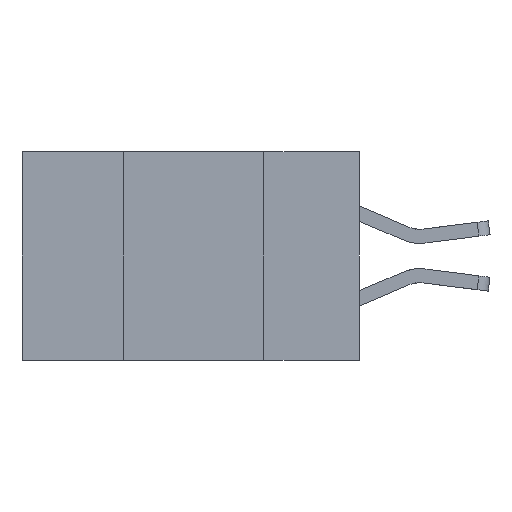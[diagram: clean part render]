
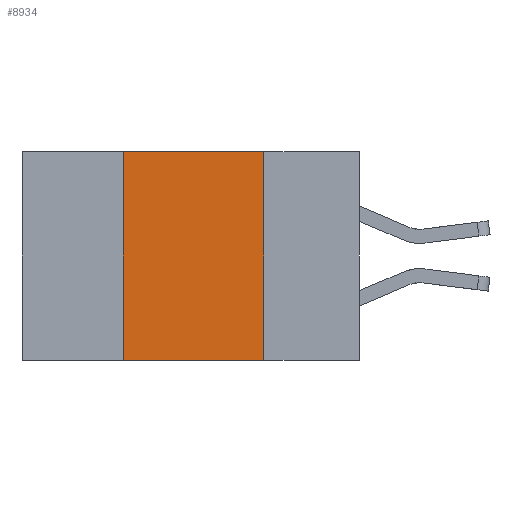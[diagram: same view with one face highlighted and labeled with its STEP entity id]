
A CAD part, left-side view. The second image highlights one B-rep face of the part: STEP entity #8934.
In plain terms, the highlighted planar face has unit normal (-1, 0, 0).
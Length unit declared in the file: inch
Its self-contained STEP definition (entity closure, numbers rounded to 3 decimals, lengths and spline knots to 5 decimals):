
#46 = CARTESIAN_POINT ( 'NONE',  ( 0., 0.42, 0. ) ) ;
#115 = CARTESIAN_POINT ( 'NONE',  ( 0., 0.17, 0. ) ) ;
#658 = CARTESIAN_POINT ( 'NONE',  ( 0., 0.42, 0. ) ) ;
#924 = PLANE ( 'NONE',  #6355 ) ;
#1428 = LINE ( 'NONE', #11579, #11336 ) ;
#2015 = CARTESIAN_POINT ( 'NONE',  ( 0., 0.6, 0. ) ) ;
#2362 = CARTESIAN_POINT ( 'NONE',  ( 0., 0.6, 0. ) ) ;
#2534 = CARTESIAN_POINT ( 'NONE',  ( 0., 0.42, -0.37 ) ) ;
#3047 = DIRECTION ( 'NONE',  ( 1., 0., 0. ) ) ;
#3139 = CARTESIAN_POINT ( 'NONE',  ( 0., 0.17, -0.37 ) ) ;
#3356 = VERTEX_POINT ( 'NONE', #2534 ) ;
#3390 = ORIENTED_EDGE ( 'NONE', *, *, #7328, .T. ) ;
#3649 = DIRECTION ( 'NONE',  ( 0., -1., 0. ) ) ;
#3976 = VERTEX_POINT ( 'NONE', #46 ) ;
#4279 = VERTEX_POINT ( 'NONE', #115 ) ;
#5111 = LINE ( 'NONE', #2362, #12308 ) ;
#5125 = ORIENTED_EDGE ( 'NONE', *, *, #9436, .F. ) ;
#5731 = ORIENTED_EDGE ( 'NONE', *, *, #11399, .F. ) ;
#5743 = DIRECTION ( 'NONE',  ( 0., 0., 1. ) ) ;
#6355 = AXIS2_PLACEMENT_3D ( 'NONE', #2015, #3047, #9742 ) ;
#6870 = FACE_OUTER_BOUND ( 'NONE', #10212, .T. ) ;
#6895 = EDGE_CURVE ( 'NONE', #3976, #4279, #5111, .T. ) ;
#7129 = VERTEX_POINT ( 'NONE', #3139 ) ;
#7328 = EDGE_CURVE ( 'NONE', #3356, #7129, #9019, .T. ) ;
#8717 = VECTOR ( 'NONE', #12482, 39.37008 ) ;
#8934 = ADVANCED_FACE ( 'NONE', ( #6870 ), #924, .F. ) ;
#9019 = LINE ( 'NONE', #11508, #8717 ) ;
#9436 = EDGE_CURVE ( 'NONE', #3356, #3976, #10376, .T. ) ;
#9742 = DIRECTION ( 'NONE',  ( 0., 0., -1. ) ) ;
#10212 = EDGE_LOOP ( 'NONE', ( #5731, #12339, #5125, #3390 ) ) ;
#10376 = LINE ( 'NONE', #658, #10968 ) ;
#10680 = DIRECTION ( 'NONE',  ( 0., 0., -1. ) ) ;
#10968 = VECTOR ( 'NONE', #5743, 39.37008 ) ;
#11336 = VECTOR ( 'NONE', #10680, 39.37008 ) ;
#11399 = EDGE_CURVE ( 'NONE', #4279, #7129, #1428, .T. ) ;
#11508 = CARTESIAN_POINT ( 'NONE',  ( 0., 0.6, -0.37 ) ) ;
#11579 = CARTESIAN_POINT ( 'NONE',  ( 0., 0.17, 0. ) ) ;
#12308 = VECTOR ( 'NONE', #3649, 39.37008 ) ;
#12339 = ORIENTED_EDGE ( 'NONE', *, *, #6895, .F. ) ;
#12482 = DIRECTION ( 'NONE',  ( 0., -1., 0. ) ) ;
